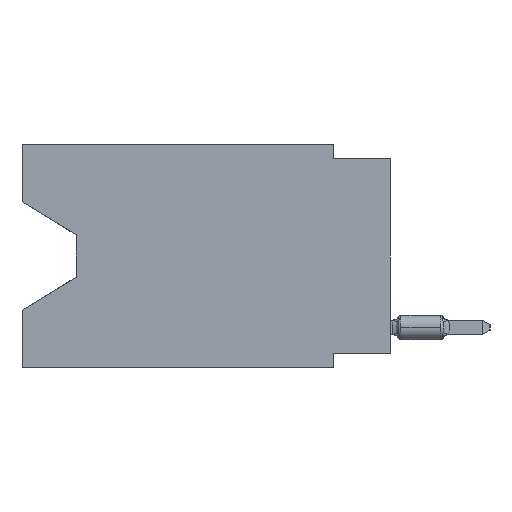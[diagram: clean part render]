
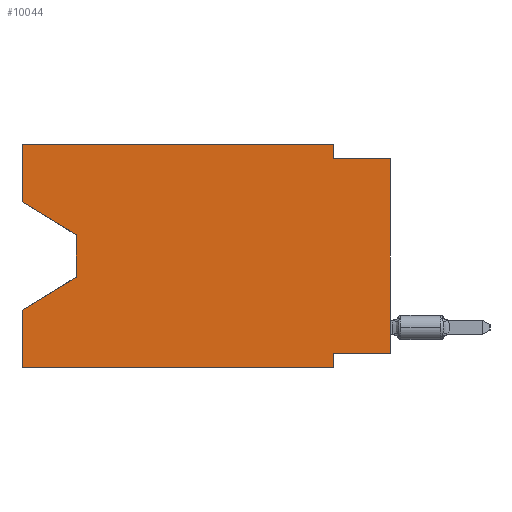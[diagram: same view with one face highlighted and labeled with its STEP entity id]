
A CAD part, left-side view. The second image highlights one B-rep face of the part: STEP entity #10044.
In plain terms, the highlighted planar face has unit normal (-1, 0, 0).
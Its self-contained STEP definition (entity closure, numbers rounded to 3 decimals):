
#667 = LINE ( 'NONE', #20639, #8697 ) ;
#868 = VECTOR ( 'NONE', #16634, 1000. ) ;
#1632 = VECTOR ( 'NONE', #10036, 1000. ) ;
#1743 = EDGE_CURVE ( 'NONE', #8184, #37071, #32994, .T. ) ;
#2076 = CARTESIAN_POINT ( 'NONE',  ( 0., 16.383, -9.906 ) ) ;
#2599 = CARTESIAN_POINT ( 'NONE',  ( 0., 0., -9.271 ) ) ;
#2666 = CARTESIAN_POINT ( 'NONE',  ( 0., 2.54, -9.906 ) ) ;
#2814 = CARTESIAN_POINT ( 'NONE',  ( 0., 2.54, 0. ) ) ;
#2937 = CARTESIAN_POINT ( 'NONE',  ( 0., 16.383, 0. ) ) ;
#2960 = CARTESIAN_POINT ( 'NONE',  ( 0., 16.383, 0. ) ) ;
#3190 = VECTOR ( 'NONE', #22608, 1000. ) ;
#3420 = VECTOR ( 'NONE', #25861, 1000. ) ;
#3589 = DIRECTION ( 'NONE',  ( 0., -1., 0. ) ) ;
#4210 = ORIENTED_EDGE ( 'NONE', *, *, #37274, .F. ) ;
#4671 = VERTEX_POINT ( 'NONE', #5536 ) ;
#5061 = ORIENTED_EDGE ( 'NONE', *, *, #12660, .T. ) ;
#5254 = VECTOR ( 'NONE', #3589, 1000. ) ;
#5536 = CARTESIAN_POINT ( 'NONE',  ( 0., 16.383, 0. ) ) ;
#6039 = CARTESIAN_POINT ( 'NONE',  ( 0., 0., -9.271 ) ) ;
#6288 = DIRECTION ( 'NONE',  ( 0., -1., 0. ) ) ;
#7835 = CARTESIAN_POINT ( 'NONE',  ( 0., 16.383, -7.36 ) ) ;
#8184 = VERTEX_POINT ( 'NONE', #32782 ) ;
#8218 = CARTESIAN_POINT ( 'NONE',  ( 0., 16.383, 0. ) ) ;
#8226 = CARTESIAN_POINT ( 'NONE',  ( 0., 2.54, -9.271 ) ) ;
#8572 = CARTESIAN_POINT ( 'NONE',  ( 0., 0., 0. ) ) ;
#8697 = VECTOR ( 'NONE', #34294, 1000. ) ;
#9828 = CARTESIAN_POINT ( 'NONE',  ( 0., 16.383, -2.546 ) ) ;
#10036 = DIRECTION ( 'NONE',  ( 0., 0.855, -0.519 ) ) ;
#10044 = ADVANCED_FACE ( 'NONE', ( #15167 ), #29512, .F. ) ;
#10064 = VECTOR ( 'NONE', #12020, 1000. ) ;
#10337 = DIRECTION ( 'NONE',  ( 0., 0., 1. ) ) ;
#10521 = EDGE_CURVE ( 'NONE', #25465, #4671, #13920, .T. ) ;
#10816 = ORIENTED_EDGE ( 'NONE', *, *, #14124, .F. ) ;
#10956 = VERTEX_POINT ( 'NONE', #2666 ) ;
#11067 = ORIENTED_EDGE ( 'NONE', *, *, #16196, .F. ) ;
#11173 = VERTEX_POINT ( 'NONE', #8226 ) ;
#12020 = DIRECTION ( 'NONE',  ( 0., -0.855, -0.519 ) ) ;
#12222 = CARTESIAN_POINT ( 'NONE',  ( 0., 13.97, -5.893 ) ) ;
#12393 = DIRECTION ( 'NONE',  ( 0., 0., 1. ) ) ;
#12660 = EDGE_CURVE ( 'NONE', #25465, #38538, #18078, .T. ) ;
#12871 = ORIENTED_EDGE ( 'NONE', *, *, #21648, .T. ) ;
#13457 = CARTESIAN_POINT ( 'NONE',  ( 0., 16.383, 0. ) ) ;
#13579 = ORIENTED_EDGE ( 'NONE', *, *, #24388, .T. ) ;
#13920 = LINE ( 'NONE', #2937, #32312 ) ;
#13959 = AXIS2_PLACEMENT_3D ( 'NONE', #8218, #32431, #42518 ) ;
#14124 = EDGE_CURVE ( 'NONE', #23914, #40816, #17250, .T. ) ;
#14251 = ORIENTED_EDGE ( 'NONE', *, *, #39073, .T. ) ;
#14836 = VERTEX_POINT ( 'NONE', #2599 ) ;
#15167 = FACE_OUTER_BOUND ( 'NONE', #31021, .T. ) ;
#15885 = LINE ( 'NONE', #6039, #18492 ) ;
#16124 = ORIENTED_EDGE ( 'NONE', *, *, #17154, .F. ) ;
#16196 = EDGE_CURVE ( 'NONE', #37108, #23914, #18344, .T. ) ;
#16634 = DIRECTION ( 'NONE',  ( 0., 0., 1. ) ) ;
#17154 = EDGE_CURVE ( 'NONE', #4671, #37108, #27163, .T. ) ;
#17250 = LINE ( 'NONE', #41882, #5254 ) ;
#18078 = LINE ( 'NONE', #32192, #10064 ) ;
#18344 = LINE ( 'NONE', #2814, #3190 ) ;
#18492 = VECTOR ( 'NONE', #23318, 1000. ) ;
#19061 = LINE ( 'NONE', #26034, #20273 ) ;
#20273 = VECTOR ( 'NONE', #32727, 1000. ) ;
#20639 = CARTESIAN_POINT ( 'NONE',  ( 0., 2.54, -9.906 ) ) ;
#21252 = ORIENTED_EDGE ( 'NONE', *, *, #30352, .F. ) ;
#21338 = VECTOR ( 'NONE', #12393, 1000. ) ;
#21648 = EDGE_CURVE ( 'NONE', #38538, #39955, #19061, .T. ) ;
#22608 = DIRECTION ( 'NONE',  ( 0., 0., -1. ) ) ;
#22670 = CARTESIAN_POINT ( 'NONE',  ( 0., 0., -0.635 ) ) ;
#22944 = LINE ( 'NONE', #8572, #21338 ) ;
#23318 = DIRECTION ( 'NONE',  ( 0., 1., 0. ) ) ;
#23914 = VERTEX_POINT ( 'NONE', #31732 ) ;
#24388 = EDGE_CURVE ( 'NONE', #8184, #10956, #37031, .T. ) ;
#25465 = VERTEX_POINT ( 'NONE', #9828 ) ;
#25861 = DIRECTION ( 'NONE',  ( 0., -1., 0. ) ) ;
#26034 = CARTESIAN_POINT ( 'NONE',  ( 0., 13.97, -4.013 ) ) ;
#27145 = ORIENTED_EDGE ( 'NONE', *, *, #33742, .T. ) ;
#27163 = LINE ( 'NONE', #13457, #42565 ) ;
#29512 = PLANE ( 'NONE',  #13959 ) ;
#30352 = EDGE_CURVE ( 'NONE', #11173, #10956, #667, .T. ) ;
#31021 = EDGE_LOOP ( 'NONE', ( #5061, #12871, #27145, #42728, #13579, #21252, #4210, #14251, #10816, #11067, #16124, #42384 ) ) ;
#31732 = CARTESIAN_POINT ( 'NONE',  ( 0., 2.54, -0.635 ) ) ;
#32192 = CARTESIAN_POINT ( 'NONE',  ( 0., 16.383, -2.546 ) ) ;
#32312 = VECTOR ( 'NONE', #10337, 1000. ) ;
#32431 = DIRECTION ( 'NONE',  ( 1., 0., 0. ) ) ;
#32705 = CARTESIAN_POINT ( 'NONE',  ( 0., 2.54, 0. ) ) ;
#32727 = DIRECTION ( 'NONE',  ( 0., 0., -1. ) ) ;
#32782 = CARTESIAN_POINT ( 'NONE',  ( 0., 16.383, -9.906 ) ) ;
#32994 = LINE ( 'NONE', #2960, #868 ) ;
#33140 = CARTESIAN_POINT ( 'NONE',  ( 0., 13.97, -5.893 ) ) ;
#33742 = EDGE_CURVE ( 'NONE', #39955, #37071, #40072, .T. ) ;
#34294 = DIRECTION ( 'NONE',  ( 0., 0., -1. ) ) ;
#37031 = LINE ( 'NONE', #2076, #3420 ) ;
#37071 = VERTEX_POINT ( 'NONE', #7835 ) ;
#37108 = VERTEX_POINT ( 'NONE', #32705 ) ;
#37178 = CARTESIAN_POINT ( 'NONE',  ( 0., 13.97, -4.013 ) ) ;
#37274 = EDGE_CURVE ( 'NONE', #14836, #11173, #15885, .T. ) ;
#38538 = VERTEX_POINT ( 'NONE', #37178 ) ;
#39073 = EDGE_CURVE ( 'NONE', #14836, #40816, #22944, .T. ) ;
#39955 = VERTEX_POINT ( 'NONE', #12222 ) ;
#40072 = LINE ( 'NONE', #33140, #1632 ) ;
#40816 = VERTEX_POINT ( 'NONE', #22670 ) ;
#41882 = CARTESIAN_POINT ( 'NONE',  ( 0., 0., -0.635 ) ) ;
#42384 = ORIENTED_EDGE ( 'NONE', *, *, #10521, .F. ) ;
#42518 = DIRECTION ( 'NONE',  ( 0., 0., -1. ) ) ;
#42565 = VECTOR ( 'NONE', #6288, 1000. ) ;
#42728 = ORIENTED_EDGE ( 'NONE', *, *, #1743, .F. ) ;
